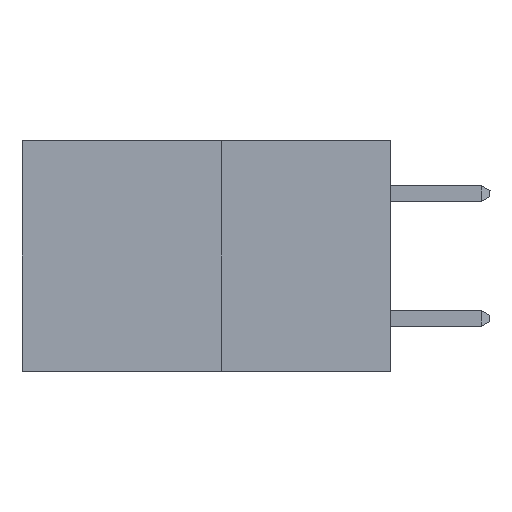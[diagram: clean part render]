
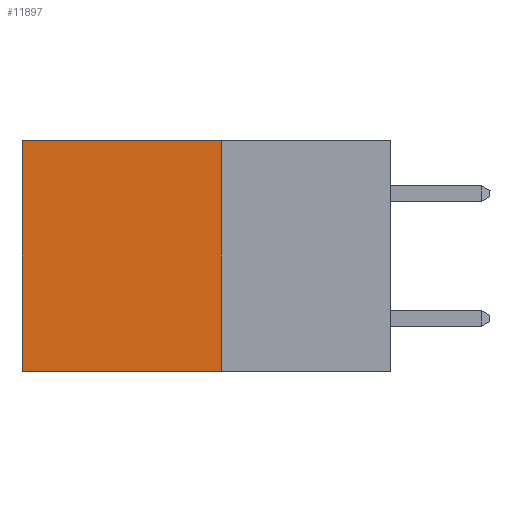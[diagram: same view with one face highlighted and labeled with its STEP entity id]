
A CAD part, left-side view. The second image highlights one B-rep face of the part: STEP entity #11897.
In plain terms, the highlighted planar face has unit normal (-1, 0, 0).
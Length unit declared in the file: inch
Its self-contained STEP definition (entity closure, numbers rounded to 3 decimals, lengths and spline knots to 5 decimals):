
#242 = VERTEX_POINT ( 'NONE', #9297 ) ;
#447 = ORIENTED_EDGE ( 'NONE', *, *, #1849, .T. ) ;
#870 = DIRECTION ( 'NONE',  ( 0., 0., -1. ) ) ;
#913 = VECTOR ( 'NONE', #10409, 39.37008 ) ;
#980 = LINE ( 'NONE', #1521, #11403 ) ;
#1035 = VECTOR ( 'NONE', #11167, 39.37008 ) ;
#1324 = FACE_OUTER_BOUND ( 'NONE', #4577, .T. ) ;
#1521 = CARTESIAN_POINT ( 'NONE',  ( 0.277, 0.27, -0.37 ) ) ;
#1660 = VERTEX_POINT ( 'NONE', #10543 ) ;
#1849 = EDGE_CURVE ( 'NONE', #1660, #12067, #4091, .T. ) ;
#1999 = LINE ( 'NONE', #10393, #913 ) ;
#3307 = CARTESIAN_POINT ( 'NONE',  ( 0.277, 0.27, 0. ) ) ;
#3467 = DIRECTION ( 'NONE',  ( 0., 1., 0. ) ) ;
#3795 = EDGE_CURVE ( 'NONE', #12067, #242, #1999, .T. ) ;
#4091 = LINE ( 'NONE', #3307, #9026 ) ;
#4577 = EDGE_LOOP ( 'NONE', ( #8171, #10728, #8465, #447 ) ) ;
#5711 = EDGE_CURVE ( 'NONE', #1660, #6851, #11449, .T. ) ;
#6100 = AXIS2_PLACEMENT_3D ( 'NONE', #6187, #7165, #870 ) ;
#6187 = CARTESIAN_POINT ( 'NONE',  ( 0.277, 0.27, -0.37 ) ) ;
#6363 = CARTESIAN_POINT ( 'NONE',  ( 0.277, 0.59, 0. ) ) ;
#6851 = VERTEX_POINT ( 'NONE', #11168 ) ;
#7165 = DIRECTION ( 'NONE',  ( 1., 0., 0. ) ) ;
#8171 = ORIENTED_EDGE ( 'NONE', *, *, #3795, .T. ) ;
#8465 = ORIENTED_EDGE ( 'NONE', *, *, #5711, .F. ) ;
#8666 = DIRECTION ( 'NONE',  ( 0., 1., 0. ) ) ;
#9026 = VECTOR ( 'NONE', #3467, 39.37008 ) ;
#9297 = CARTESIAN_POINT ( 'NONE',  ( 0.277, 0.59, -0.37 ) ) ;
#10393 = CARTESIAN_POINT ( 'NONE',  ( 0.277, 0.59, -0.37 ) ) ;
#10409 = DIRECTION ( 'NONE',  ( 0., 0., -1. ) ) ;
#10543 = CARTESIAN_POINT ( 'NONE',  ( 0.277, 0.27, 0. ) ) ;
#10728 = ORIENTED_EDGE ( 'NONE', *, *, #10992, .F. ) ;
#10992 = EDGE_CURVE ( 'NONE', #6851, #242, #980, .T. ) ;
#11167 = DIRECTION ( 'NONE',  ( 0., 0., -1. ) ) ;
#11168 = CARTESIAN_POINT ( 'NONE',  ( 0.277, 0.27, -0.37 ) ) ;
#11232 = CARTESIAN_POINT ( 'NONE',  ( 0.277, 0.27, -0.37 ) ) ;
#11403 = VECTOR ( 'NONE', #8666, 39.37008 ) ;
#11449 = LINE ( 'NONE', #11232, #1035 ) ;
#11897 = ADVANCED_FACE ( 'NONE', ( #1324 ), #11942, .F. ) ;
#11942 = PLANE ( 'NONE',  #6100 ) ;
#12067 = VERTEX_POINT ( 'NONE', #6363 ) ;
